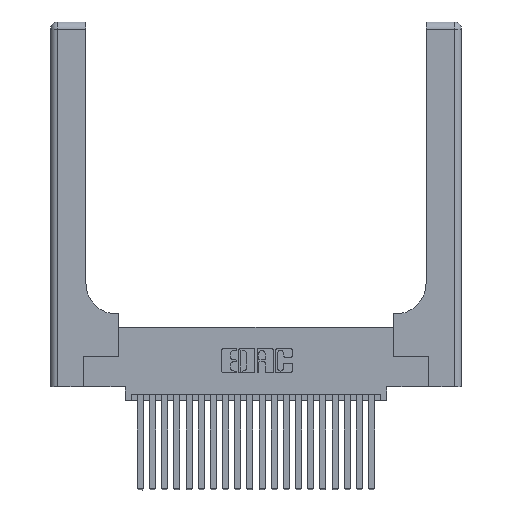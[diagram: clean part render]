
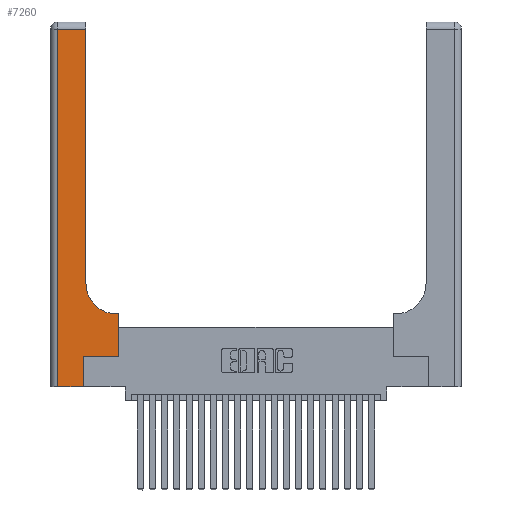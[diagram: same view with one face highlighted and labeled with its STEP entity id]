
A CAD part, top view. The second image highlights one B-rep face of the part: STEP entity #7260.
In plain terms, the highlighted planar face has unit normal (0, 0, 1).
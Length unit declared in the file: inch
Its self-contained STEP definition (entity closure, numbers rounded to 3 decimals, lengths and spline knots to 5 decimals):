
#151 = DIRECTION ( 'NONE',  ( 0., 1., 0. ) ) ;
#389 = CARTESIAN_POINT ( 'NONE',  ( 0.5415, 0.85, 0.37 ) ) ;
#519 = AXIS2_PLACEMENT_3D ( 'NONE', #389, #18700, #2162 ) ;
#1116 = EDGE_CURVE ( 'NONE', #23606, #12354, #15753, .T. ) ;
#2162 = DIRECTION ( 'NONE',  ( 1., 0., 0. ) ) ;
#2359 = EDGE_CURVE ( 'NONE', #20588, #7755, #14545, .T. ) ;
#2761 = CARTESIAN_POINT ( 'NONE',  ( 0., 3., 0.37 ) ) ;
#3649 = VERTEX_POINT ( 'NONE', #16780 ) ;
#3812 = CARTESIAN_POINT ( 'NONE',  ( 0.2915, 0.85, 0.37 ) ) ;
#3927 = VECTOR ( 'NONE', #18889, 39.37008 ) ;
#4208 = CARTESIAN_POINT ( 'NONE',  ( 0., 2.94, 0.37 ) ) ;
#4536 = EDGE_CURVE ( 'NONE', #12354, #21244, #15588, .T. ) ;
#4586 = ORIENTED_EDGE ( 'NONE', *, *, #23293, .T. ) ;
#4625 = DIRECTION ( 'NONE',  ( 0., 0., -1. ) ) ;
#4762 = CARTESIAN_POINT ( 'NONE',  ( 0.5415, 0.6, 0.37 ) ) ;
#4843 = VECTOR ( 'NONE', #13264, 39.37008 ) ;
#5000 = CARTESIAN_POINT ( 'NONE',  ( 0.269, 0.25, 0.37 ) ) ;
#6044 = AXIS2_PLACEMENT_3D ( 'NONE', #2761, #4625, #11997 ) ;
#6148 = ORIENTED_EDGE ( 'NONE', *, *, #4536, .T. ) ;
#6852 = CARTESIAN_POINT ( 'NONE',  ( 0.06, 2.94, 0.37 ) ) ;
#7032 = ORIENTED_EDGE ( 'NONE', *, *, #12064, .T. ) ;
#7260 = ADVANCED_FACE ( 'NONE', ( #10901 ), #23092, .F. ) ;
#7696 = CARTESIAN_POINT ( 'NONE',  ( 0.269, 0., 0.37 ) ) ;
#7755 = VERTEX_POINT ( 'NONE', #8194 ) ;
#7782 = VERTEX_POINT ( 'NONE', #4762 ) ;
#7938 = ORIENTED_EDGE ( 'NONE', *, *, #1116, .T. ) ;
#7987 = DIRECTION ( 'NONE',  ( -1., 0., 0. ) ) ;
#8194 = CARTESIAN_POINT ( 'NONE',  ( 0.2915, 2.94, 0.37 ) ) ;
#8673 = CARTESIAN_POINT ( 'NONE',  ( 0., 0., 0.37 ) ) ;
#10179 = VECTOR ( 'NONE', #20336, 39.37008 ) ;
#10724 = VECTOR ( 'NONE', #15821, 39.37008 ) ;
#10830 = VECTOR ( 'NONE', #19628, 39.37008 ) ;
#10854 = EDGE_LOOP ( 'NONE', ( #13982, #4586, #7938, #6148, #12260, #23386, #22923, #7032, #16912 ) ) ;
#10901 = FACE_OUTER_BOUND ( 'NONE', #10854, .T. ) ;
#11997 = DIRECTION ( 'NONE',  ( -1., 0., 0. ) ) ;
#12064 = EDGE_CURVE ( 'NONE', #23042, #7782, #16532, .T. ) ;
#12260 = ORIENTED_EDGE ( 'NONE', *, *, #17756, .T. ) ;
#12354 = VERTEX_POINT ( 'NONE', #18687 ) ;
#13264 = DIRECTION ( 'NONE',  ( 0., -1., 0. ) ) ;
#13917 = CARTESIAN_POINT ( 'NONE',  ( 0.2915, 0.6, 0.37 ) ) ;
#13982 = ORIENTED_EDGE ( 'NONE', *, *, #2359, .T. ) ;
#14095 = CARTESIAN_POINT ( 'NONE',  ( 0.2915, 3., 0.37 ) ) ;
#14545 = LINE ( 'NONE', #14095, #10830 ) ;
#14773 = VECTOR ( 'NONE', #17983, 39.37008 ) ;
#15187 = CARTESIAN_POINT ( 'NONE',  ( 0.269, 0.25, 0.37 ) ) ;
#15588 = LINE ( 'NONE', #8673, #10724 ) ;
#15749 = CIRCLE ( 'NONE', #519, 0.25 ) ;
#15753 = LINE ( 'NONE', #18654, #4843 ) ;
#15821 = DIRECTION ( 'NONE',  ( 1., 0., 0. ) ) ;
#16532 = LINE ( 'NONE', #13917, #14773 ) ;
#16549 = CARTESIAN_POINT ( 'NONE',  ( 0.5585, 0.25, 0.37 ) ) ;
#16780 = CARTESIAN_POINT ( 'NONE',  ( 0.5585, 0.25, 0.37 ) ) ;
#16912 = ORIENTED_EDGE ( 'NONE', *, *, #21102, .T. ) ;
#17714 = VECTOR ( 'NONE', #7987, 39.37008 ) ;
#17756 = EDGE_CURVE ( 'NONE', #21244, #22718, #19086, .T. ) ;
#17983 = DIRECTION ( 'NONE',  ( -1., 0., 0. ) ) ;
#18654 = CARTESIAN_POINT ( 'NONE',  ( 0.06, 3., 0.37 ) ) ;
#18687 = CARTESIAN_POINT ( 'NONE',  ( 0.06, 0., 0.37 ) ) ;
#18700 = DIRECTION ( 'NONE',  ( 0., 0., -1. ) ) ;
#18889 = DIRECTION ( 'NONE',  ( 1., 0., 0. ) ) ;
#19086 = LINE ( 'NONE', #19812, #10179 ) ;
#19628 = DIRECTION ( 'NONE',  ( 0., 1., 0. ) ) ;
#19812 = CARTESIAN_POINT ( 'NONE',  ( 0.269, 0., 0.37 ) ) ;
#20336 = DIRECTION ( 'NONE',  ( 0., 1., 0. ) ) ;
#20352 = CARTESIAN_POINT ( 'NONE',  ( 0.5585, 0.6, 0.37 ) ) ;
#20588 = VERTEX_POINT ( 'NONE', #3812 ) ;
#21102 = EDGE_CURVE ( 'NONE', #7782, #20588, #15749, .T. ) ;
#21185 = EDGE_CURVE ( 'NONE', #3649, #23042, #23568, .T. ) ;
#21244 = VERTEX_POINT ( 'NONE', #7696 ) ;
#21779 = VECTOR ( 'NONE', #151, 39.37008 ) ;
#22718 = VERTEX_POINT ( 'NONE', #5000 ) ;
#22874 = LINE ( 'NONE', #15187, #3927 ) ;
#22923 = ORIENTED_EDGE ( 'NONE', *, *, #21185, .T. ) ;
#23042 = VERTEX_POINT ( 'NONE', #20352 ) ;
#23092 = PLANE ( 'NONE',  #6044 ) ;
#23293 = EDGE_CURVE ( 'NONE', #7755, #23606, #23483, .T. ) ;
#23386 = ORIENTED_EDGE ( 'NONE', *, *, #23431, .T. ) ;
#23431 = EDGE_CURVE ( 'NONE', #22718, #3649, #22874, .T. ) ;
#23483 = LINE ( 'NONE', #4208, #17714 ) ;
#23568 = LINE ( 'NONE', #16549, #21779 ) ;
#23606 = VERTEX_POINT ( 'NONE', #6852 ) ;
